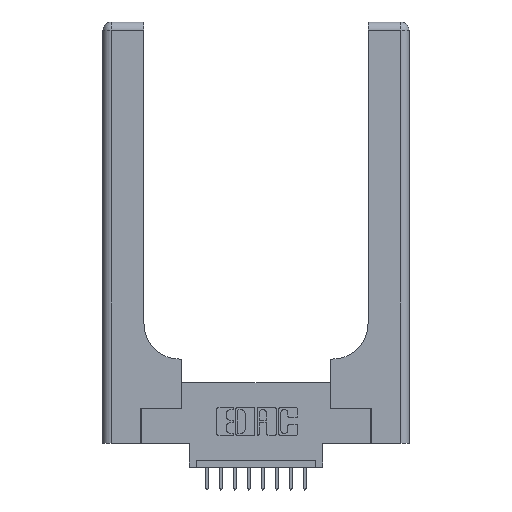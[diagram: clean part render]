
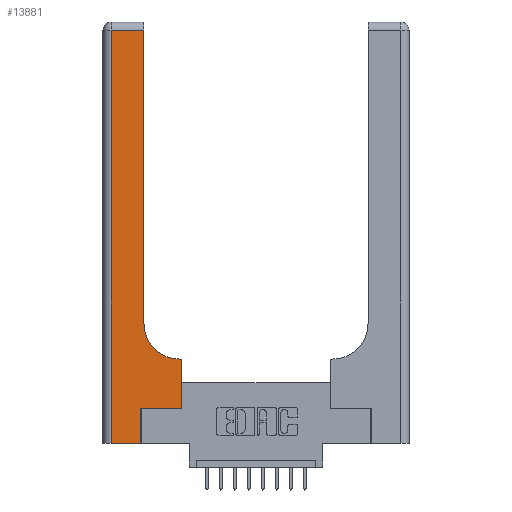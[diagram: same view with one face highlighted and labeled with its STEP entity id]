
A CAD part, top view. The second image highlights one B-rep face of the part: STEP entity #13881.
In plain terms, the highlighted planar face has unit normal (0, 0, 1).
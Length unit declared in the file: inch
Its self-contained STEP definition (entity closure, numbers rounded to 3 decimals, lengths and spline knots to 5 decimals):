
#128 = CARTESIAN_POINT ( 'NONE',  ( 0.5585, 0.6, 0.37 ) ) ;
#234 = LINE ( 'NONE', #11113, #1406 ) ;
#731 = ORIENTED_EDGE ( 'NONE', *, *, #9107, .T. ) ;
#1065 = CARTESIAN_POINT ( 'NONE',  ( 0.5585, 0.25, 0.37 ) ) ;
#1071 = DIRECTION ( 'NONE',  ( 0., 1., 0. ) ) ;
#1168 = PLANE ( 'NONE',  #2554 ) ;
#1406 = VECTOR ( 'NONE', #6175, 39.37008 ) ;
#1449 = ORIENTED_EDGE ( 'NONE', *, *, #11804, .T. ) ;
#1510 = LINE ( 'NONE', #2734, #6892 ) ;
#1643 = VERTEX_POINT ( 'NONE', #4772 ) ;
#2297 = DIRECTION ( 'NONE',  ( 0., 0., -1. ) ) ;
#2458 = CARTESIAN_POINT ( 'NONE',  ( 0.269, 0.25, 0.37 ) ) ;
#2554 = AXIS2_PLACEMENT_3D ( 'NONE', #11033, #2297, #12330 ) ;
#2672 = DIRECTION ( 'NONE',  ( 0., -1., 0. ) ) ;
#2734 = CARTESIAN_POINT ( 'NONE',  ( 0.06, 3., 0.37 ) ) ;
#3188 = DIRECTION ( 'NONE',  ( 0., 0., -1. ) ) ;
#4046 = VERTEX_POINT ( 'NONE', #128 ) ;
#4047 = VERTEX_POINT ( 'NONE', #8677 ) ;
#4295 = LINE ( 'NONE', #14687, #4877 ) ;
#4458 = FACE_OUTER_BOUND ( 'NONE', #4559, .T. ) ;
#4559 = EDGE_LOOP ( 'NONE', ( #731, #6253, #14510, #9334, #1449, #10963, #7649, #7400, #11105 ) ) ;
#4567 = EDGE_CURVE ( 'NONE', #4046, #4047, #15805, .T. ) ;
#4772 = CARTESIAN_POINT ( 'NONE',  ( 0.06, 2.94, 0.37 ) ) ;
#4877 = VECTOR ( 'NONE', #7257, 39.37008 ) ;
#5054 = CARTESIAN_POINT ( 'NONE',  ( 0., 2.94, 0.37 ) ) ;
#5480 = CARTESIAN_POINT ( 'NONE',  ( 0.2915, 3., 0.37 ) ) ;
#5601 = VECTOR ( 'NONE', #9681, 39.37008 ) ;
#5713 = VERTEX_POINT ( 'NONE', #12433 ) ;
#5937 = VECTOR ( 'NONE', #15396, 39.37008 ) ;
#6038 = DIRECTION ( 'NONE',  ( -1., 0., 0. ) ) ;
#6175 = DIRECTION ( 'NONE',  ( 1., 0., 0. ) ) ;
#6253 = ORIENTED_EDGE ( 'NONE', *, *, #12746, .T. ) ;
#6632 = LINE ( 'NONE', #5054, #9526 ) ;
#6892 = VECTOR ( 'NONE', #2672, 39.37008 ) ;
#7153 = CARTESIAN_POINT ( 'NONE',  ( 0.2915, 2.94, 0.37 ) ) ;
#7200 = EDGE_CURVE ( 'NONE', #4047, #5713, #12261, .T. ) ;
#7257 = DIRECTION ( 'NONE',  ( 1., 0., 0. ) ) ;
#7400 = ORIENTED_EDGE ( 'NONE', *, *, #4567, .T. ) ;
#7413 = VECTOR ( 'NONE', #1071, 39.37008 ) ;
#7649 = ORIENTED_EDGE ( 'NONE', *, *, #15981, .T. ) ;
#7930 = VERTEX_POINT ( 'NONE', #9151 ) ;
#8022 = CARTESIAN_POINT ( 'NONE',  ( 0.5415, 0.85, 0.37 ) ) ;
#8677 = CARTESIAN_POINT ( 'NONE',  ( 0.5415, 0.6, 0.37 ) ) ;
#8893 = LINE ( 'NONE', #1065, #5601 ) ;
#9107 = EDGE_CURVE ( 'NONE', #5713, #10398, #15055, .T. ) ;
#9151 = CARTESIAN_POINT ( 'NONE',  ( 0.269, 0., 0.37 ) ) ;
#9334 = ORIENTED_EDGE ( 'NONE', *, *, #13319, .T. ) ;
#9526 = VECTOR ( 'NONE', #14858, 39.37008 ) ;
#9681 = DIRECTION ( 'NONE',  ( 0., 1., 0. ) ) ;
#9708 = VERTEX_POINT ( 'NONE', #11894 ) ;
#10398 = VERTEX_POINT ( 'NONE', #7153 ) ;
#10615 = EDGE_CURVE ( 'NONE', #1643, #14445, #1510, .T. ) ;
#10926 = CARTESIAN_POINT ( 'NONE',  ( 0.2915, 0.6, 0.37 ) ) ;
#10941 = CARTESIAN_POINT ( 'NONE',  ( 0.269, 0., 0.37 ) ) ;
#10963 = ORIENTED_EDGE ( 'NONE', *, *, #15430, .T. ) ;
#11033 = CARTESIAN_POINT ( 'NONE',  ( 0., 3., 0.37 ) ) ;
#11105 = ORIENTED_EDGE ( 'NONE', *, *, #7200, .T. ) ;
#11113 = CARTESIAN_POINT ( 'NONE',  ( 0.269, 0.25, 0.37 ) ) ;
#11380 = CARTESIAN_POINT ( 'NONE',  ( 0.06, 0., 0.37 ) ) ;
#11699 = LINE ( 'NONE', #10941, #7413 ) ;
#11804 = EDGE_CURVE ( 'NONE', #7930, #13387, #11699, .T. ) ;
#11894 = CARTESIAN_POINT ( 'NONE',  ( 0.5585, 0.25, 0.37 ) ) ;
#12261 = CIRCLE ( 'NONE', #16009, 0.25 ) ;
#12330 = DIRECTION ( 'NONE',  ( -1., 0., 0. ) ) ;
#12433 = CARTESIAN_POINT ( 'NONE',  ( 0.2915, 0.85, 0.37 ) ) ;
#12746 = EDGE_CURVE ( 'NONE', #10398, #1643, #6632, .T. ) ;
#12980 = DIRECTION ( 'NONE',  ( 1., 0., 0. ) ) ;
#13096 = VECTOR ( 'NONE', #6038, 39.37008 ) ;
#13319 = EDGE_CURVE ( 'NONE', #14445, #7930, #4295, .T. ) ;
#13387 = VERTEX_POINT ( 'NONE', #2458 ) ;
#13881 = ADVANCED_FACE ( 'NONE', ( #4458 ), #1168, .F. ) ;
#14445 = VERTEX_POINT ( 'NONE', #11380 ) ;
#14510 = ORIENTED_EDGE ( 'NONE', *, *, #10615, .T. ) ;
#14687 = CARTESIAN_POINT ( 'NONE',  ( 0., 0., 0.37 ) ) ;
#14858 = DIRECTION ( 'NONE',  ( -1., 0., 0. ) ) ;
#15055 = LINE ( 'NONE', #5480, #5937 ) ;
#15396 = DIRECTION ( 'NONE',  ( 0., 1., 0. ) ) ;
#15430 = EDGE_CURVE ( 'NONE', #13387, #9708, #234, .T. ) ;
#15805 = LINE ( 'NONE', #10926, #13096 ) ;
#15981 = EDGE_CURVE ( 'NONE', #9708, #4046, #8893, .T. ) ;
#16009 = AXIS2_PLACEMENT_3D ( 'NONE', #8022, #3188, #12980 ) ;
